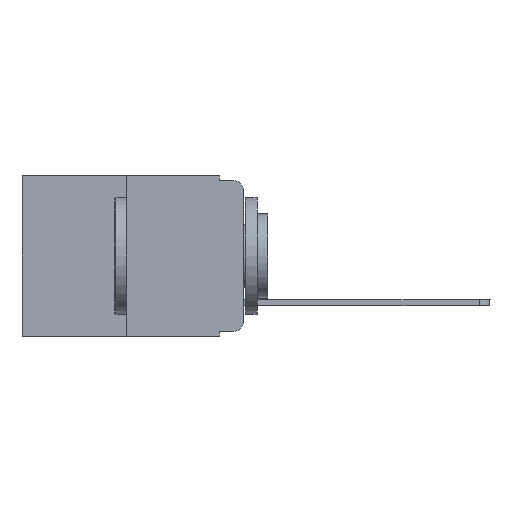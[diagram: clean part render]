
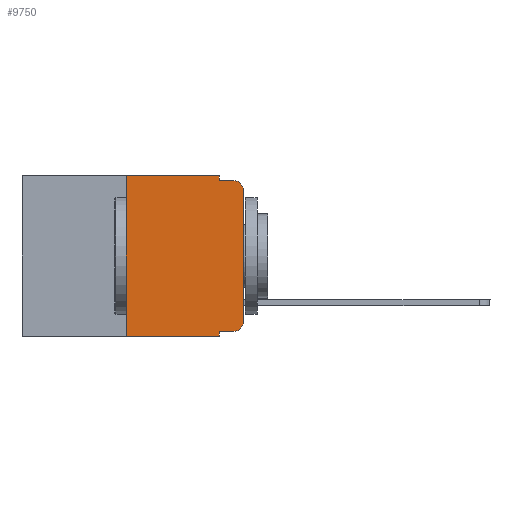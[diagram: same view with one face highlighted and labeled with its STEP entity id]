
A CAD part, left-side view. The second image highlights one B-rep face of the part: STEP entity #9750.
In plain terms, the highlighted planar face has unit normal (-1, 0, 0).
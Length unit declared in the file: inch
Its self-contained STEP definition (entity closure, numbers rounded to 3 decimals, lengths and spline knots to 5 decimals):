
#101 = ORIENTED_EDGE ( 'NONE', *, *, #7164, .F. ) ;
#530 = EDGE_CURVE ( 'NONE', #4291, #13120, #12665, .T. ) ;
#571 = CARTESIAN_POINT ( 'NONE',  ( 0., 0.051, -0.333 ) ) ;
#822 = CARTESIAN_POINT ( 'NONE',  ( 0., 0.051, -0.343 ) ) ;
#1045 = VECTOR ( 'NONE', #9260, 39.37008 ) ;
#1311 = PLANE ( 'NONE',  #10117 ) ;
#1399 = DIRECTION ( 'NONE',  ( 0., 0., -1. ) ) ;
#2352 = CIRCLE ( 'NONE', #2644, 0.02 ) ;
#2379 = CARTESIAN_POINT ( 'NONE',  ( 0., 0.473, 0. ) ) ;
#2558 = DIRECTION ( 'NONE',  ( 1., 0., 0. ) ) ;
#2644 = AXIS2_PLACEMENT_3D ( 'NONE', #14982, #9311, #9487 ) ;
#2662 = EDGE_LOOP ( 'NONE', ( #3375, #9976, #101, #6128, #17782, #5799, #13901, #2721, #16363, #14452 ) ) ;
#2721 = ORIENTED_EDGE ( 'NONE', *, *, #13330, .F. ) ;
#2913 = VERTEX_POINT ( 'NONE', #16255 ) ;
#3198 = CARTESIAN_POINT ( 'NONE',  ( 0., 0.02, -0.01 ) ) ;
#3375 = ORIENTED_EDGE ( 'NONE', *, *, #4983, .T. ) ;
#3388 = CARTESIAN_POINT ( 'NONE',  ( 0., 0.25, 0. ) ) ;
#3679 = CARTESIAN_POINT ( 'NONE',  ( 0., 0.051, -0.01 ) ) ;
#3948 = DIRECTION ( 'NONE',  ( 0., 0., -1. ) ) ;
#4112 = LINE ( 'NONE', #6954, #9527 ) ;
#4291 = VERTEX_POINT ( 'NONE', #7576 ) ;
#4806 = VECTOR ( 'NONE', #12698, 39.37008 ) ;
#4983 = EDGE_CURVE ( 'NONE', #13120, #18660, #8449, .T. ) ;
#5434 = VECTOR ( 'NONE', #3948, 39.37008 ) ;
#5764 = CARTESIAN_POINT ( 'NONE',  ( 0., 0.02, -0.313 ) ) ;
#5799 = ORIENTED_EDGE ( 'NONE', *, *, #17846, .F. ) ;
#5896 = CARTESIAN_POINT ( 'NONE',  ( 0., 0., -0.03 ) ) ;
#6093 = CARTESIAN_POINT ( 'NONE',  ( 0., 0.051, -0.01 ) ) ;
#6128 = ORIENTED_EDGE ( 'NONE', *, *, #14216, .F. ) ;
#6340 = DIRECTION ( 'NONE',  ( 0., -1., 0. ) ) ;
#6954 = CARTESIAN_POINT ( 'NONE',  ( 0., 0.473, -0.343 ) ) ;
#7164 = EDGE_CURVE ( 'NONE', #15112, #16521, #15207, .T. ) ;
#7518 = VERTEX_POINT ( 'NONE', #9048 ) ;
#7576 = CARTESIAN_POINT ( 'NONE',  ( 0., 0.02, -0.333 ) ) ;
#7670 = VECTOR ( 'NONE', #9243, 39.37008 ) ;
#7751 = EDGE_CURVE ( 'NONE', #2913, #12959, #4112, .T. ) ;
#7894 = LINE ( 'NONE', #15172, #11295 ) ;
#8274 = LINE ( 'NONE', #11039, #5434 ) ;
#8449 = LINE ( 'NONE', #9883, #8852 ) ;
#8561 = VERTEX_POINT ( 'NONE', #18692 ) ;
#8852 = VECTOR ( 'NONE', #15643, 39.37008 ) ;
#9048 = CARTESIAN_POINT ( 'NONE',  ( 0., 0.051, 0. ) ) ;
#9203 = EDGE_CURVE ( 'NONE', #18660, #16521, #2352, .T. ) ;
#9243 = DIRECTION ( 'NONE',  ( 0., 0., 1. ) ) ;
#9260 = DIRECTION ( 'NONE',  ( 0., -1., 0. ) ) ;
#9311 = DIRECTION ( 'NONE',  ( -1., 0., 0. ) ) ;
#9487 = DIRECTION ( 'NONE',  ( 0., 0., -1. ) ) ;
#9527 = VECTOR ( 'NONE', #14041, 39.37008 ) ;
#9594 = DIRECTION ( 'NONE',  ( 0., -1., 0. ) ) ;
#9750 = ADVANCED_FACE ( 'NONE', ( #15502 ), #1311, .F. ) ;
#9883 = CARTESIAN_POINT ( 'NONE',  ( 0., 0., 0. ) ) ;
#9976 = ORIENTED_EDGE ( 'NONE', *, *, #9203, .T. ) ;
#10117 = AXIS2_PLACEMENT_3D ( 'NONE', #2379, #2558, #14187 ) ;
#10266 = CARTESIAN_POINT ( 'NONE',  ( 0., 0.051, -0.333 ) ) ;
#11039 = CARTESIAN_POINT ( 'NONE',  ( 0., 0.051, 0. ) ) ;
#11295 = VECTOR ( 'NONE', #9594, 39.37008 ) ;
#11377 = VERTEX_POINT ( 'NONE', #10266 ) ;
#12507 = VECTOR ( 'NONE', #6340, 39.37008 ) ;
#12665 = CIRCLE ( 'NONE', #16580, 0.02 ) ;
#12698 = DIRECTION ( 'NONE',  ( 0., 0., -1. ) ) ;
#12959 = VERTEX_POINT ( 'NONE', #822 ) ;
#13120 = VERTEX_POINT ( 'NONE', #17169 ) ;
#13330 = EDGE_CURVE ( 'NONE', #11377, #12959, #14106, .T. ) ;
#13531 = LINE ( 'NONE', #571, #12507 ) ;
#13901 = ORIENTED_EDGE ( 'NONE', *, *, #7751, .T. ) ;
#14041 = DIRECTION ( 'NONE',  ( 0., -1., 0. ) ) ;
#14106 = LINE ( 'NONE', #15341, #4806 ) ;
#14187 = DIRECTION ( 'NONE',  ( 0., 0., -1. ) ) ;
#14216 = EDGE_CURVE ( 'NONE', #7518, #15112, #8274, .T. ) ;
#14452 = ORIENTED_EDGE ( 'NONE', *, *, #530, .T. ) ;
#14982 = CARTESIAN_POINT ( 'NONE',  ( 0., 0.02, -0.03 ) ) ;
#15112 = VERTEX_POINT ( 'NONE', #6093 ) ;
#15172 = CARTESIAN_POINT ( 'NONE',  ( 0., 0.473, 0. ) ) ;
#15207 = LINE ( 'NONE', #3679, #1045 ) ;
#15341 = CARTESIAN_POINT ( 'NONE',  ( 0., 0.051, 0. ) ) ;
#15502 = FACE_OUTER_BOUND ( 'NONE', #2662, .T. ) ;
#15643 = DIRECTION ( 'NONE',  ( 0., 0., 1. ) ) ;
#16150 = DIRECTION ( 'NONE',  ( -1., 0., 0. ) ) ;
#16159 = EDGE_CURVE ( 'NONE', #11377, #4291, #13531, .T. ) ;
#16255 = CARTESIAN_POINT ( 'NONE',  ( 0., 0.25, -0.343 ) ) ;
#16338 = LINE ( 'NONE', #3388, #7670 ) ;
#16363 = ORIENTED_EDGE ( 'NONE', *, *, #16159, .T. ) ;
#16521 = VERTEX_POINT ( 'NONE', #3198 ) ;
#16580 = AXIS2_PLACEMENT_3D ( 'NONE', #5764, #16150, #1399 ) ;
#17169 = CARTESIAN_POINT ( 'NONE',  ( 0., 0., -0.313 ) ) ;
#17782 = ORIENTED_EDGE ( 'NONE', *, *, #18445, .F. ) ;
#17846 = EDGE_CURVE ( 'NONE', #2913, #8561, #16338, .T. ) ;
#18445 = EDGE_CURVE ( 'NONE', #8561, #7518, #7894, .T. ) ;
#18660 = VERTEX_POINT ( 'NONE', #5896 ) ;
#18692 = CARTESIAN_POINT ( 'NONE',  ( 0., 0.25, 0. ) ) ;
